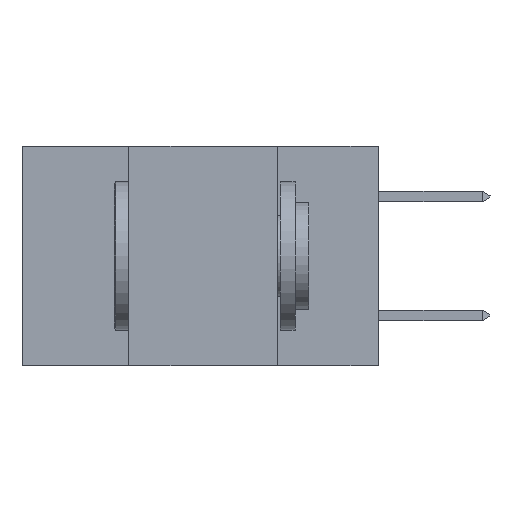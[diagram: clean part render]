
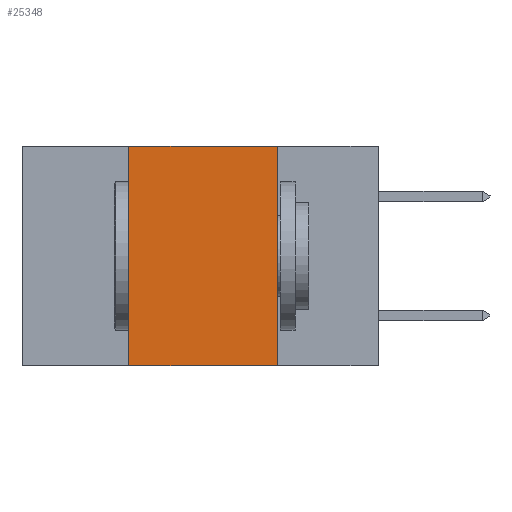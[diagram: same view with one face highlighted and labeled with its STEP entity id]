
A CAD part, left-side view. The second image highlights one B-rep face of the part: STEP entity #25348.
In plain terms, the highlighted planar face has unit normal (-1, 0, 0).
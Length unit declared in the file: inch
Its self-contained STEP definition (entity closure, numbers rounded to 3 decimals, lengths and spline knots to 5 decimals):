
#989 = CARTESIAN_POINT ( 'NONE',  ( 0., 0.42, -0.37 ) ) ;
#1128 = DIRECTION ( 'NONE',  ( 0., 0., -1. ) ) ;
#1568 = CARTESIAN_POINT ( 'NONE',  ( 0., 0.6, -0.37 ) ) ;
#2149 = DIRECTION ( 'NONE',  ( 0., -1., 0. ) ) ;
#2439 = CARTESIAN_POINT ( 'NONE',  ( 0., 0.42, -0.37 ) ) ;
#2859 = LINE ( 'NONE', #989, #5866 ) ;
#2968 = EDGE_CURVE ( 'NONE', #17423, #23673, #17724, .T. ) ;
#4887 = DIRECTION ( 'NONE',  ( 0., 0., -1. ) ) ;
#5162 = ORIENTED_EDGE ( 'NONE', *, *, #26943, .T. ) ;
#5866 = VECTOR ( 'NONE', #22774, 39.37008 ) ;
#7188 = CARTESIAN_POINT ( 'NONE',  ( 0., 0.17, -0.37 ) ) ;
#7902 = DIRECTION ( 'NONE',  ( 0., -1., 0. ) ) ;
#8686 = ORIENTED_EDGE ( 'NONE', *, *, #12749, .F. ) ;
#9704 = VECTOR ( 'NONE', #2149, 39.37008 ) ;
#9708 = ORIENTED_EDGE ( 'NONE', *, *, #12766, .F. ) ;
#9789 = FACE_OUTER_BOUND ( 'NONE', #14326, .T. ) ;
#11412 = VECTOR ( 'NONE', #1128, 39.37008 ) ;
#12361 = CARTESIAN_POINT ( 'NONE',  ( 0., 0.17, -0.37 ) ) ;
#12749 = EDGE_CURVE ( 'NONE', #23847, #17423, #2859, .T. ) ;
#12766 = EDGE_CURVE ( 'NONE', #23673, #12881, #20614, .T. ) ;
#12881 = VERTEX_POINT ( 'NONE', #12361 ) ;
#13945 = VECTOR ( 'NONE', #7902, 39.37008 ) ;
#14326 = EDGE_LOOP ( 'NONE', ( #9708, #15713, #8686, #5162 ) ) ;
#15511 = CARTESIAN_POINT ( 'NONE',  ( 0., 0.42, 0. ) ) ;
#15713 = ORIENTED_EDGE ( 'NONE', *, *, #2968, .F. ) ;
#15844 = DIRECTION ( 'NONE',  ( 1., 0., 0. ) ) ;
#16405 = AXIS2_PLACEMENT_3D ( 'NONE', #18604, #15844, #4887 ) ;
#17423 = VERTEX_POINT ( 'NONE', #15511 ) ;
#17724 = LINE ( 'NONE', #24219, #9704 ) ;
#18604 = CARTESIAN_POINT ( 'NONE',  ( 0., 0.6, 0. ) ) ;
#19307 = LINE ( 'NONE', #1568, #13945 ) ;
#20614 = LINE ( 'NONE', #7188, #11412 ) ;
#22500 = PLANE ( 'NONE',  #16405 ) ;
#22774 = DIRECTION ( 'NONE',  ( 0., 0., 1. ) ) ;
#23378 = CARTESIAN_POINT ( 'NONE',  ( 0., 0.17, 0. ) ) ;
#23673 = VERTEX_POINT ( 'NONE', #23378 ) ;
#23847 = VERTEX_POINT ( 'NONE', #2439 ) ;
#24219 = CARTESIAN_POINT ( 'NONE',  ( 0., 0.6, 0. ) ) ;
#25348 = ADVANCED_FACE ( 'NONE', ( #9789 ), #22500, .F. ) ;
#26943 = EDGE_CURVE ( 'NONE', #23847, #12881, #19307, .T. ) ;
